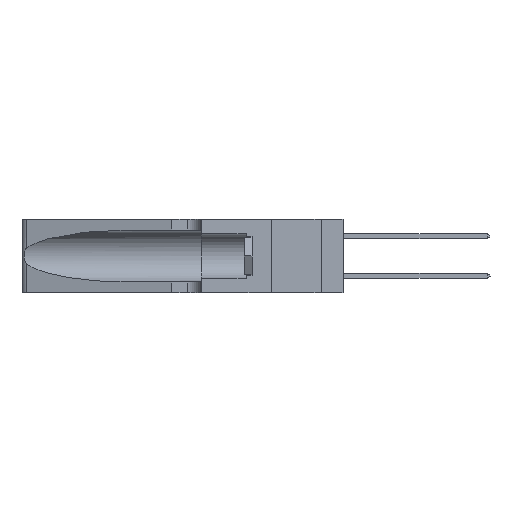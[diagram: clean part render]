
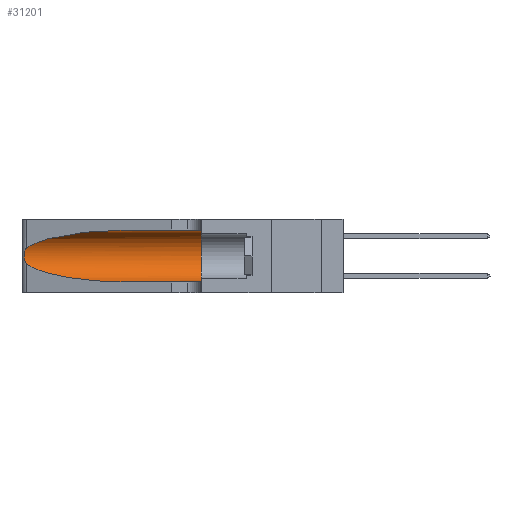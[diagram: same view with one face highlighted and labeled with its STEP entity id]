
A CAD part, left-side view. The second image highlights one B-rep face of the part: STEP entity #31201.
In plain terms, the highlighted cylindrical face has radius 3.308 mm (diameter 6.617 mm), a partial arc.
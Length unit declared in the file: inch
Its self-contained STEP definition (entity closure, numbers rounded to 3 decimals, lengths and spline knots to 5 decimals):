
#79 = CARTESIAN_POINT ( 'NONE',  ( 0.18966, 0.96281, 0.31525 ) ) ;
#1649 = VERTEX_POINT ( 'NONE', #35950 ) ;
#2158 = CARTESIAN_POINT ( 'NONE',  ( 0.2373, 1.15595, 0.28018 ) ) ;
#2398 = EDGE_CURVE ( 'NONE', #9340, #21801, #17734, .T. ) ;
#2461 = ORIENTED_EDGE ( 'NONE', *, *, #35570, .F. ) ;
#2500 = VERTEX_POINT ( 'NONE', #10486 ) ;
#3297 = CARTESIAN_POINT ( 'NONE',  ( 0.25854, 1.2359, 0.20912 ) ) ;
#3302 = VERTEX_POINT ( 'NONE', #28933 ) ;
#3509 = ORIENTED_EDGE ( 'NONE', *, *, #2398, .T. ) ;
#3555 = CARTESIAN_POINT ( 'NONE',  ( 0.25487, 1.22718, 0.22369 ) ) ;
#5736 = ORIENTED_EDGE ( 'NONE', *, *, #37003, .T. ) ;
#6347 = CARTESIAN_POINT ( 'NONE',  ( 0.26075, 1.23896, 0.178 ) ) ;
#8269 = CARTESIAN_POINT ( 'NONE',  ( 0.1305, 1.61858, 0.05475 ) ) ;
#8801 = VECTOR ( 'NONE', #26483, 39.37008 ) ;
#9275 = CARTESIAN_POINT ( 'NONE',  ( 0.25856, 1.23593, 0.16098 ) ) ;
#9340 = VERTEX_POINT ( 'NONE', #36362 ) ;
#10486 = CARTESIAN_POINT ( 'NONE',  ( 0.25487, 1.22718, 0.14631 ) ) ;
#10487 = CARTESIAN_POINT ( 'NONE',  ( 0.1305, 1.61858, 0.31525 ) ) ;
#11322 = EDGE_CURVE ( 'NONE', #22696, #21801, #22150, .T. ) ;
#12146 = CARTESIAN_POINT ( 'NONE',  ( 0.25639, 1.23184, 0.21858 ) ) ;
#12393 = CARTESIAN_POINT ( 'NONE',  ( 0.26075, 1.23896, 0.19203 ) ) ;
#13134 = DIRECTION ( 'NONE',  ( 0., -1., 0. ) ) ;
#14447 = CARTESIAN_POINT ( 'NONE',  ( 0.1305, 0.72297, 0.05475 ) ) ;
#16306 = CARTESIAN_POINT ( 'NONE',  ( 0.1305, 1.61858, 0.185 ) ) ;
#17224 = CARTESIAN_POINT ( 'NONE',  ( 0.1305, 0.35, 0.05475 ) ) ;
#17734 = LINE ( 'NONE', #8269, #8801 ) ;
#18124 = ORIENTED_EDGE ( 'NONE', *, *, #11322, .F. ) ;
#18207 = CARTESIAN_POINT ( 'NONE',  ( 0.25789, 1.23486, 0.15765 ) ) ;
#18442 = DIRECTION ( 'NONE',  ( 0., 0., 1. ) ) ;
#21607 = CARTESIAN_POINT ( 'NONE',  ( 0.25555, 1.22993, 0.14849 ) ) ;
#21801 = VERTEX_POINT ( 'NONE', #17224 ) ;
#21982 = AXIS2_PLACEMENT_3D ( 'NONE', #16306, #31545, #34472 ) ;
#22150 = CIRCLE ( 'NONE', #33709, 0.13025 ) ;
#22696 = VERTEX_POINT ( 'NONE', #30419 ) ;
#23056 = CARTESIAN_POINT ( 'NONE',  ( 0.2373, 1.15595, 0.08982 ) ) ;
#24412 = DIRECTION ( 'NONE',  ( 0., 1., 0. ) ) ;
#25246 = LINE ( 'NONE', #10487, #29060 ) ;
#26483 = DIRECTION ( 'NONE',  ( 0., -1., 0. ) ) ;
#27362 = CARTESIAN_POINT ( 'NONE',  ( 0.25487, 1.22718, 0.14631 ) ) ;
#27711 = CARTESIAN_POINT ( 'NONE',  ( 0.1305, 0.72297, 0.31525 ) ) ;
#27728 = CARTESIAN_POINT ( 'NONE',  ( 0.26017, 1.23833, 0.17102 ) ) ;
#28933 = CARTESIAN_POINT ( 'NONE',  ( 0.25487, 1.22718, 0.22369 ) ) ;
#29060 = VECTOR ( 'NONE', #13134, 39.37008 ) ;
#29359 = EDGE_LOOP ( 'NONE', ( #36920, #5736, #33287, #3509, #18124, #2461 ) ) ;
#30273 = CARTESIAN_POINT ( 'NONE',  ( 0.25555, 1.22994, 0.2215 ) ) ;
#30419 = CARTESIAN_POINT ( 'NONE',  ( 0.1305, 0.35, 0.31525 ) ) ;
#30775 = CARTESIAN_POINT ( 'NONE',  ( 0.26018, 1.23835, 0.19895 ) ) ;
#31201 = ADVANCED_FACE ( 'NONE', ( #32691 ), #36996, .F. ) ;
#31467 = EDGE_CURVE ( 'NONE', #2500, #9340, #38696, .T. ) ;
#31545 = DIRECTION ( 'NONE',  ( 0., -1., 0. ) ) ;
#32691 = FACE_OUTER_BOUND ( 'NONE', #29359, .T. ) ;
#33058 = EDGE_CURVE ( 'NONE', #1649, #3302, #35050, .T. ) ;
#33287 = ORIENTED_EDGE ( 'NONE', *, *, #31467, .T. ) ;
#33294 = CARTESIAN_POINT ( 'NONE',  ( 0.25639, 1.23186, 0.15144 ) ) ;
#33412 = CARTESIAN_POINT ( 'NONE',  ( 0.1305, 0.35, 0.185 ) ) ;
#33709 = AXIS2_PLACEMENT_3D ( 'NONE', #33412, #24412, #18442 ) ;
#33831 = CARTESIAN_POINT ( 'NONE',  ( 0.25787, 1.23484, 0.2124 ) ) ;
#34472 = DIRECTION ( 'NONE',  ( 0., 0., -1. ) ) ;
#35050 =( BOUNDED_CURVE ( )  B_SPLINE_CURVE ( 3, ( #27711, #79, #2158, #36406 ),
 .UNSPECIFIED., .F., .F. ) 
 B_SPLINE_CURVE_WITH_KNOTS ( ( 4, 4 ),
 ( 1.5708, 2.84003 ),
 .UNSPECIFIED. ) 
 CURVE ( )  GEOMETRIC_REPRESENTATION_ITEM ( )  RATIONAL_B_SPLINE_CURVE ( ( 1., 0.87, 0.87, 1. ) ) 
 REPRESENTATION_ITEM ( '' )  );
#35570 = EDGE_CURVE ( 'NONE', #1649, #22696, #25246, .T. ) ;
#35950 = CARTESIAN_POINT ( 'NONE',  ( 0.1305, 0.72297, 0.31525 ) ) ;
#36362 = CARTESIAN_POINT ( 'NONE',  ( 0.1305, 0.72297, 0.05475 ) ) ;
#36406 = CARTESIAN_POINT ( 'NONE',  ( 0.25487, 1.22718, 0.22369 ) ) ;
#36920 = ORIENTED_EDGE ( 'NONE', *, *, #33058, .T. ) ;
#36996 = CYLINDRICAL_SURFACE ( 'NONE', #21982, 0.13025 ) ;
#37003 = EDGE_CURVE ( 'NONE', #3302, #2500, #38215, .T. ) ;
#38200 = CARTESIAN_POINT ( 'NONE',  ( 0.25487, 1.22718, 0.14631 ) ) ;
#38215 = B_SPLINE_CURVE_WITH_KNOTS ( 'NONE', 3,
 ( #3555, #30273, #12146, #33831, #3297, #30775, #12393, #6347, #27728, #9275, #18207, #33294, #21607, #27362 ),
 .UNSPECIFIED., .F., .F.,
 ( 4, 2, 2, 2, 2, 2, 4 ),
 ( 0., 0.00027, 0.00053, 0.00107, 0.0016, 0.00187, 0.00214 ),
 .UNSPECIFIED. ) ;
#38696 =( BOUNDED_CURVE ( )  B_SPLINE_CURVE ( 3, ( #38200, #23056, #38845, #14447 ),
 .UNSPECIFIED., .F., .T. ) 
 B_SPLINE_CURVE_WITH_KNOTS ( ( 4, 4 ),
 ( 3.44316, 4.71239 ),
 .UNSPECIFIED. ) 
 CURVE ( )  GEOMETRIC_REPRESENTATION_ITEM ( )  RATIONAL_B_SPLINE_CURVE ( ( 1., 0.87, 0.87, 1. ) ) 
 REPRESENTATION_ITEM ( '' )  );
#38845 = CARTESIAN_POINT ( 'NONE',  ( 0.18966, 0.96281, 0.05475 ) ) ;
